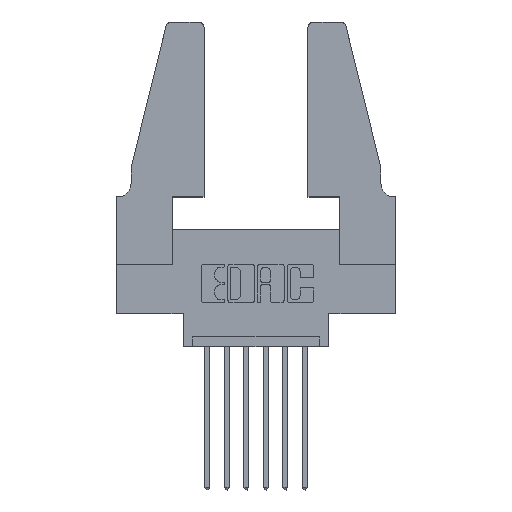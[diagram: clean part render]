
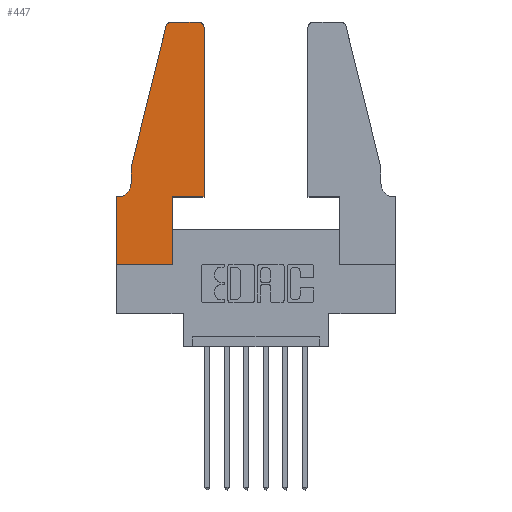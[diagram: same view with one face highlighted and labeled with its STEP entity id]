
A CAD part, top view. The second image highlights one B-rep face of the part: STEP entity #447.
In plain terms, the highlighted planar face has unit normal (0, 0, 1).
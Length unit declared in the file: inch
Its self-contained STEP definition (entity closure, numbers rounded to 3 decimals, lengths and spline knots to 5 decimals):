
#304 = FACE_OUTER_BOUND ( 'NONE', #587, .T. ) ;
#326 = CARTESIAN_POINT ( 'NONE',  ( 0.0755, 0.5, 0.37 ) ) ;
#447 = ADVANCED_FACE ( 'NONE', ( #304 ), #10596, .T. ) ;
#464 = VECTOR ( 'NONE', #5534, 39.37008 ) ;
#519 = VERTEX_POINT ( 'NONE', #2669 ) ;
#587 = EDGE_LOOP ( 'NONE', ( #10103, #10172, #6641, #2121, #10179, #9531, #6507, #7751, #8263, #8558, #1037, #2490 ) ) ;
#681 = CARTESIAN_POINT ( 'NONE',  ( 0.4205, 1.22, 0.37 ) ) ;
#707 = CARTESIAN_POINT ( 'NONE',  ( 0.2865, 0.35, 0.37 ) ) ;
#830 = VECTOR ( 'NONE', #3552, 39.37008 ) ;
#942 = VERTEX_POINT ( 'NONE', #707 ) ;
#962 = CARTESIAN_POINT ( 'NONE',  ( 0., 0., 0.37 ) ) ;
#1037 = ORIENTED_EDGE ( 'NONE', *, *, #8306, .T. ) ;
#1073 = EDGE_CURVE ( 'NONE', #942, #8374, #11283, .T. ) ;
#1107 = EDGE_CURVE ( 'NONE', #1627, #7934, #3520, .T. ) ;
#1627 = VERTEX_POINT ( 'NONE', #4373 ) ;
#1764 = CARTESIAN_POINT ( 'NONE',  ( 0.4505, 0.35, 0.37 ) ) ;
#2121 = ORIENTED_EDGE ( 'NONE', *, *, #11034, .T. ) ;
#2184 = EDGE_CURVE ( 'NONE', #6531, #4898, #5874, .T. ) ;
#2196 = VERTEX_POINT ( 'NONE', #10508 ) ;
#2235 = EDGE_CURVE ( 'NONE', #3036, #5598, #7157, .T. ) ;
#2490 = ORIENTED_EDGE ( 'NONE', *, *, #2184, .T. ) ;
#2517 = CARTESIAN_POINT ( 'NONE',  ( 0., 0.35, 0.37 ) ) ;
#2540 = CARTESIAN_POINT ( 'NONE',  ( 0., 0.35, 0.37 ) ) ;
#2669 = CARTESIAN_POINT ( 'NONE',  ( 0.284, 1.25, 0.37 ) ) ;
#3036 = VERTEX_POINT ( 'NONE', #962 ) ;
#3185 = VECTOR ( 'NONE', #9972, 39.37008 ) ;
#3401 = CARTESIAN_POINT ( 'NONE',  ( 0.284, 1.22, 0.37 ) ) ;
#3520 = LINE ( 'NONE', #8104, #10855 ) ;
#3552 = DIRECTION ( 'NONE',  ( 0., 1., 0. ) ) ;
#3699 = CARTESIAN_POINT ( 'NONE',  ( 0.4505, 0.35, 0.37 ) ) ;
#3916 = DIRECTION ( 'NONE',  ( -1., 0., 0. ) ) ;
#4218 = VECTOR ( 'NONE', #8337, 39.37008 ) ;
#4262 = LINE ( 'NONE', #9138, #464 ) ;
#4346 = DIRECTION ( 'NONE',  ( 1., 0., 0. ) ) ;
#4350 = CARTESIAN_POINT ( 'NONE',  ( 0.0055, 0.35, 0.37 ) ) ;
#4373 = CARTESIAN_POINT ( 'NONE',  ( 0.25487, 1.22718, 0.37 ) ) ;
#4595 = EDGE_CURVE ( 'NONE', #5056, #9664, #5554, .T. ) ;
#4898 = VERTEX_POINT ( 'NONE', #7118 ) ;
#5056 = VERTEX_POINT ( 'NONE', #4350 ) ;
#5534 = DIRECTION ( 'NONE',  ( 0., -1., 0. ) ) ;
#5554 = LINE ( 'NONE', #5691, #10917 ) ;
#5593 = AXIS2_PLACEMENT_3D ( 'NONE', #8743, #6959, #11520 ) ;
#5598 = VERTEX_POINT ( 'NONE', #5855 ) ;
#5691 = CARTESIAN_POINT ( 'NONE',  ( 0.0755, 0.35, 0.37 ) ) ;
#5855 = CARTESIAN_POINT ( 'NONE',  ( 0.2865, 0., 0.37 ) ) ;
#5874 = CIRCLE ( 'NONE', #7446, 0.03 ) ;
#5956 = DIRECTION ( 'NONE',  ( -1., 0., 0. ) ) ;
#6006 = EDGE_CURVE ( 'NONE', #9664, #3036, #10723, .T. ) ;
#6086 = DIRECTION ( 'NONE',  ( 0., 0., 1. ) ) ;
#6506 = AXIS2_PLACEMENT_3D ( 'NONE', #2517, #8001, #7086 ) ;
#6507 = ORIENTED_EDGE ( 'NONE', *, *, #6006, .T. ) ;
#6531 = VERTEX_POINT ( 'NONE', #11083 ) ;
#6542 = CIRCLE ( 'NONE', #9684, 0.03 ) ;
#6641 = ORIENTED_EDGE ( 'NONE', *, *, #1107, .T. ) ;
#6959 = DIRECTION ( 'NONE',  ( 0., 0., -1. ) ) ;
#6969 = DIRECTION ( 'NONE',  ( 0., 0., 1. ) ) ;
#6993 = DIRECTION ( 'NONE',  ( 1., 0., 0. ) ) ;
#7048 = DIRECTION ( 'NONE',  ( 1., 0., 0. ) ) ;
#7086 = DIRECTION ( 'NONE',  ( 1., 0., 0. ) ) ;
#7118 = CARTESIAN_POINT ( 'NONE',  ( 0.4205, 1.25, 0.37 ) ) ;
#7155 = LINE ( 'NONE', #7344, #830 ) ;
#7157 = LINE ( 'NONE', #11638, #3185 ) ;
#7213 = VECTOR ( 'NONE', #11058, 39.37008 ) ;
#7344 = CARTESIAN_POINT ( 'NONE',  ( 0.4505, 0.35, 0.37 ) ) ;
#7446 = AXIS2_PLACEMENT_3D ( 'NONE', #681, #6969, #7048 ) ;
#7739 = CARTESIAN_POINT ( 'NONE',  ( 0.2605, 1.25, 0.37 ) ) ;
#7751 = ORIENTED_EDGE ( 'NONE', *, *, #2235, .T. ) ;
#7934 = VERTEX_POINT ( 'NONE', #326 ) ;
#8001 = DIRECTION ( 'NONE',  ( 0., 0., 1. ) ) ;
#8104 = CARTESIAN_POINT ( 'NONE',  ( 0.0755, 0.5, 0.37 ) ) ;
#8247 = VECTOR ( 'NONE', #5956, 39.37008 ) ;
#8263 = ORIENTED_EDGE ( 'NONE', *, *, #11568, .T. ) ;
#8306 = EDGE_CURVE ( 'NONE', #8374, #6531, #7155, .T. ) ;
#8337 = DIRECTION ( 'NONE',  ( 0., -1., 0. ) ) ;
#8374 = VERTEX_POINT ( 'NONE', #3699 ) ;
#8413 = CARTESIAN_POINT ( 'NONE',  ( 0., 0., 0.37 ) ) ;
#8558 = ORIENTED_EDGE ( 'NONE', *, *, #1073, .T. ) ;
#8665 = CARTESIAN_POINT ( 'NONE',  ( 0.2865, 0.35, 0.37 ) ) ;
#8743 = CARTESIAN_POINT ( 'NONE',  ( 0.0055, 0.42, 0.37 ) ) ;
#9109 = CIRCLE ( 'NONE', #5593, 0.07 ) ;
#9138 = CARTESIAN_POINT ( 'NONE',  ( 0.0755, 0.5, 0.37 ) ) ;
#9514 = EDGE_CURVE ( 'NONE', #4898, #519, #10351, .T. ) ;
#9531 = ORIENTED_EDGE ( 'NONE', *, *, #4595, .T. ) ;
#9645 = EDGE_CURVE ( 'NONE', #519, #1627, #6542, .T. ) ;
#9664 = VERTEX_POINT ( 'NONE', #2540 ) ;
#9684 = AXIS2_PLACEMENT_3D ( 'NONE', #3401, #6086, #6993 ) ;
#9728 = EDGE_CURVE ( 'NONE', #2196, #5056, #9109, .T. ) ;
#9876 = VECTOR ( 'NONE', #4346, 39.37008 ) ;
#9972 = DIRECTION ( 'NONE',  ( 1., 0., 0. ) ) ;
#10103 = ORIENTED_EDGE ( 'NONE', *, *, #9514, .T. ) ;
#10172 = ORIENTED_EDGE ( 'NONE', *, *, #9645, .T. ) ;
#10179 = ORIENTED_EDGE ( 'NONE', *, *, #9728, .T. ) ;
#10351 = LINE ( 'NONE', #7739, #8247 ) ;
#10508 = CARTESIAN_POINT ( 'NONE',  ( 0.0755, 0.42, 0.37 ) ) ;
#10596 = PLANE ( 'NONE',  #6506 ) ;
#10723 = LINE ( 'NONE', #8413, #4218 ) ;
#10855 = VECTOR ( 'NONE', #11661, 39.37008 ) ;
#10917 = VECTOR ( 'NONE', #3916, 39.37008 ) ;
#11009 = LINE ( 'NONE', #8665, #7213 ) ;
#11034 = EDGE_CURVE ( 'NONE', #7934, #2196, #4262, .T. ) ;
#11058 = DIRECTION ( 'NONE',  ( 0., 1., 0. ) ) ;
#11083 = CARTESIAN_POINT ( 'NONE',  ( 0.4505, 1.22, 0.37 ) ) ;
#11283 = LINE ( 'NONE', #1764, #9876 ) ;
#11520 = DIRECTION ( 'NONE',  ( -1., 0., 0. ) ) ;
#11568 = EDGE_CURVE ( 'NONE', #5598, #942, #11009, .T. ) ;
#11638 = CARTESIAN_POINT ( 'NONE',  ( 0., 0., 0.37 ) ) ;
#11661 = DIRECTION ( 'NONE',  ( -0.239, -0.971, 0. ) ) ;
